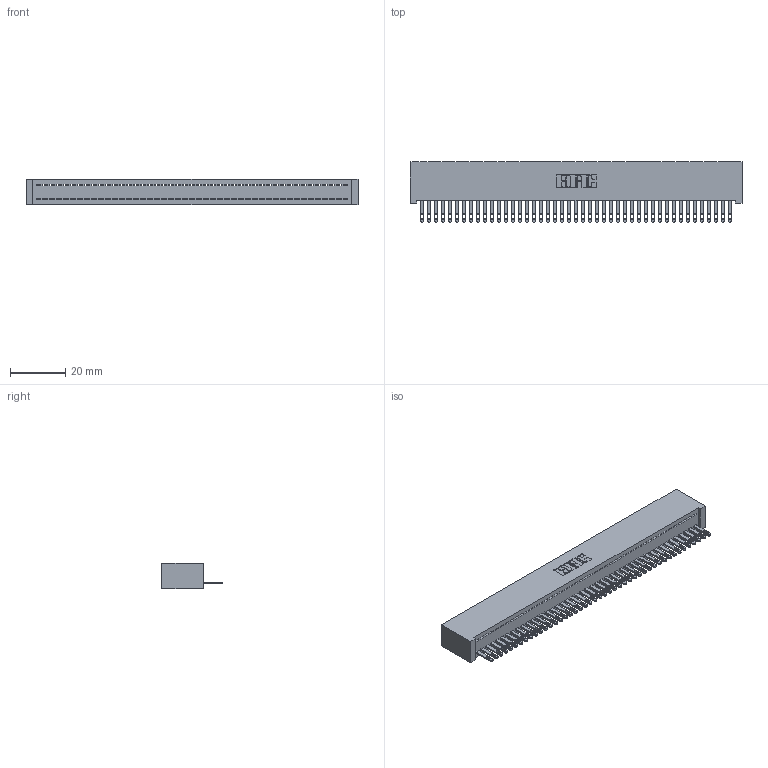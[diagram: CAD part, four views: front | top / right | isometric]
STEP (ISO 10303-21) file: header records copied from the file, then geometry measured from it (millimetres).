
FILE_DESCRIPTION (( 'STEP AP203' ), '1' );
FILE_NAME ('892-045-500-101.STEP', '2020-09-21T17:04:46', ( '' ), ( '' ), 'SwSTEP 2.0', 'SolidWorks 2020', '' );
FILE_SCHEMA (( 'CONFIG_CONTROL_DESIGN' ));
Length unit declared in the file: inch
Products named in the file (3): 345-292-001_345-293-100; 892-045-500-101; 842 Part_Lugless
Assembly tree (46 placements, depth 2):
  892-045-500-101
    842 Part_Lugless
    345-292-001_345-293-100  x45
Bounding box: 120.55 x 21.85 x 9.4 mm (x, y, z)
Volume: 11017.6 mm3; surface area: 16646.7 mm2
Topology: 46 solids, 46 shells, 2532 faces, 7835 edges, 5222 vertices
Faces by surface type: plane 1682, cylinder 850
Entity records: 26643 total; most frequent: CARTESIAN_POINT 4601, ORIENTED_EDGE 4582, DIRECTION 3869, EDGE_CURVE 2291, LINE 2167, VECTOR 2167, VERTEX_POINT 1526, AXIS2_PLACEMENT_3D 851
